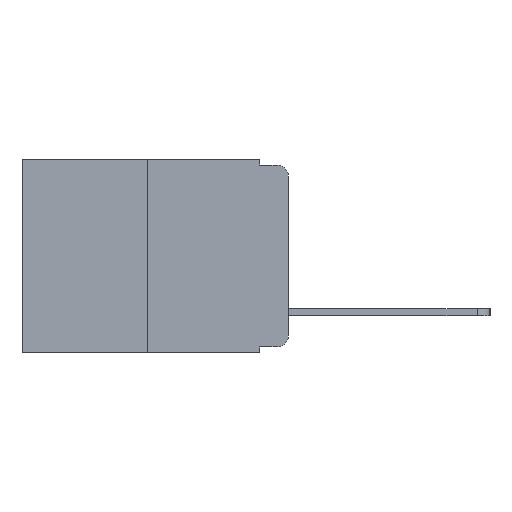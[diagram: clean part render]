
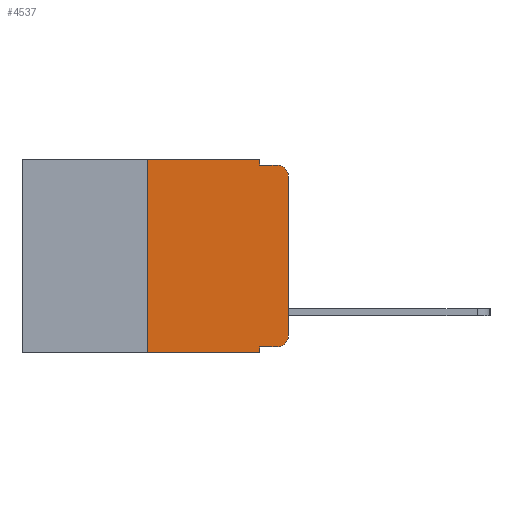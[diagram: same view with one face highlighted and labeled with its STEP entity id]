
A CAD part, left-side view. The second image highlights one B-rep face of the part: STEP entity #4537.
In plain terms, the highlighted planar face has unit normal (-1, 0, 0).
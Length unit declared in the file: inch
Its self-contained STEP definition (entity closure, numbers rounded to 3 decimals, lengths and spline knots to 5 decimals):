
#17 = CIRCLE ( 'NONE', #20758, 0.02 ) ;
#32 = VECTOR ( 'NONE', #8358, 39.37008 ) ;
#76 = DIRECTION ( 'NONE',  ( 0., -1., 0. ) ) ;
#261 = ORIENTED_EDGE ( 'NONE', *, *, #6416, .F. ) ;
#351 = VERTEX_POINT ( 'NONE', #8157 ) ;
#473 = VERTEX_POINT ( 'NONE', #11344 ) ;
#594 = CARTESIAN_POINT ( 'NONE',  ( 0., 0.051, 0. ) ) ;
#611 = AXIS2_PLACEMENT_3D ( 'NONE', #16874, #18416, #2044 ) ;
#669 = EDGE_CURVE ( 'NONE', #13733, #17383, #20309, .T. ) ;
#855 = CARTESIAN_POINT ( 'NONE',  ( 0., 0.25, 0. ) ) ;
#950 = DIRECTION ( 'NONE',  ( 0., 0., -1. ) ) ;
#1012 = VECTOR ( 'NONE', #12440, 39.37008 ) ;
#1279 = DIRECTION ( 'NONE',  ( 0., 0., -1. ) ) ;
#1845 = EDGE_CURVE ( 'NONE', #11778, #13733, #11550, .T. ) ;
#1929 = VERTEX_POINT ( 'NONE', #855 ) ;
#2044 = DIRECTION ( 'NONE',  ( 0., 0., -1. ) ) ;
#2176 = LINE ( 'NONE', #3964, #19258 ) ;
#2352 = DIRECTION ( 'NONE',  ( 0., -1., 0. ) ) ;
#2441 = VECTOR ( 'NONE', #18248, 39.37008 ) ;
#2777 = VECTOR ( 'NONE', #8556, 39.37008 ) ;
#2995 = VERTEX_POINT ( 'NONE', #15507 ) ;
#3964 = CARTESIAN_POINT ( 'NONE',  ( 0., 0.473, 0. ) ) ;
#4117 = EDGE_CURVE ( 'NONE', #11778, #473, #20318, .T. ) ;
#4208 = VECTOR ( 'NONE', #19559, 39.37008 ) ;
#4537 = ADVANCED_FACE ( 'NONE', ( #6743 ), #11356, .F. ) ;
#4577 = CARTESIAN_POINT ( 'NONE',  ( 0., 0.051, -0.01 ) ) ;
#5256 = EDGE_CURVE ( 'NONE', #351, #1929, #19521, .T. ) ;
#5560 = CARTESIAN_POINT ( 'NONE',  ( 0., 0.02, -0.333 ) ) ;
#5897 = CARTESIAN_POINT ( 'NONE',  ( 0., 0.051, 0. ) ) ;
#6416 = EDGE_CURVE ( 'NONE', #6516, #15698, #13912, .T. ) ;
#6516 = VERTEX_POINT ( 'NONE', #5897 ) ;
#6570 = VECTOR ( 'NONE', #76, 39.37008 ) ;
#6717 = EDGE_CURVE ( 'NONE', #351, #473, #8777, .T. ) ;
#6743 = FACE_OUTER_BOUND ( 'NONE', #13322, .T. ) ;
#6989 = ORIENTED_EDGE ( 'NONE', *, *, #1845, .T. ) ;
#8157 = CARTESIAN_POINT ( 'NONE',  ( 0., 0.25, -0.343 ) ) ;
#8338 = ORIENTED_EDGE ( 'NONE', *, *, #10920, .T. ) ;
#8358 = DIRECTION ( 'NONE',  ( 0., 0., 1. ) ) ;
#8556 = DIRECTION ( 'NONE',  ( 0., 0., -1. ) ) ;
#8717 = CARTESIAN_POINT ( 'NONE',  ( 0., 0.051, -0.01 ) ) ;
#8723 = EDGE_CURVE ( 'NONE', #15698, #11528, #13543, .T. ) ;
#8777 = LINE ( 'NONE', #21177, #4208 ) ;
#8848 = ORIENTED_EDGE ( 'NONE', *, *, #9826, .T. ) ;
#9166 = VECTOR ( 'NONE', #17813, 39.37008 ) ;
#9778 = CARTESIAN_POINT ( 'NONE',  ( 0., 0.473, 0. ) ) ;
#9826 = EDGE_CURVE ( 'NONE', #2995, #11528, #17, .T. ) ;
#10920 = EDGE_CURVE ( 'NONE', #17383, #2995, #12518, .T. ) ;
#11129 = DIRECTION ( 'NONE',  ( -1., 0., 0. ) ) ;
#11344 = CARTESIAN_POINT ( 'NONE',  ( 0., 0.051, -0.343 ) ) ;
#11356 = PLANE ( 'NONE',  #12160 ) ;
#11428 = DIRECTION ( 'NONE',  ( 1., 0., 0. ) ) ;
#11439 = ORIENTED_EDGE ( 'NONE', *, *, #669, .T. ) ;
#11528 = VERTEX_POINT ( 'NONE', #19815 ) ;
#11550 = LINE ( 'NONE', #17686, #6570 ) ;
#11778 = VERTEX_POINT ( 'NONE', #12328 ) ;
#12160 = AXIS2_PLACEMENT_3D ( 'NONE', #9778, #11428, #1279 ) ;
#12328 = CARTESIAN_POINT ( 'NONE',  ( 0., 0.051, -0.333 ) ) ;
#12440 = DIRECTION ( 'NONE',  ( 0., 0., -1. ) ) ;
#12518 = LINE ( 'NONE', #18091, #32 ) ;
#13238 = ORIENTED_EDGE ( 'NONE', *, *, #8723, .F. ) ;
#13322 = EDGE_LOOP ( 'NONE', ( #8338, #8848, #13238, #261, #14235, #18499, #14735, #19007, #6989, #11439 ) ) ;
#13543 = LINE ( 'NONE', #4577, #9166 ) ;
#13733 = VERTEX_POINT ( 'NONE', #5560 ) ;
#13912 = LINE ( 'NONE', #594, #1012 ) ;
#14235 = ORIENTED_EDGE ( 'NONE', *, *, #17984, .F. ) ;
#14735 = ORIENTED_EDGE ( 'NONE', *, *, #6717, .T. ) ;
#15124 = CARTESIAN_POINT ( 'NONE',  ( 0., 0.051, 0. ) ) ;
#15507 = CARTESIAN_POINT ( 'NONE',  ( 0., 0., -0.03 ) ) ;
#15698 = VERTEX_POINT ( 'NONE', #8717 ) ;
#16629 = CARTESIAN_POINT ( 'NONE',  ( 0., 0.25, 0. ) ) ;
#16874 = CARTESIAN_POINT ( 'NONE',  ( 0., 0.02, -0.313 ) ) ;
#17158 = CARTESIAN_POINT ( 'NONE',  ( 0., 0., -0.313 ) ) ;
#17383 = VERTEX_POINT ( 'NONE', #17158 ) ;
#17686 = CARTESIAN_POINT ( 'NONE',  ( 0., 0.051, -0.333 ) ) ;
#17813 = DIRECTION ( 'NONE',  ( 0., -1., 0. ) ) ;
#17984 = EDGE_CURVE ( 'NONE', #1929, #6516, #2176, .T. ) ;
#18091 = CARTESIAN_POINT ( 'NONE',  ( 0., 0., 0. ) ) ;
#18248 = DIRECTION ( 'NONE',  ( 0., 0., 1. ) ) ;
#18416 = DIRECTION ( 'NONE',  ( -1., 0., 0. ) ) ;
#18499 = ORIENTED_EDGE ( 'NONE', *, *, #5256, .F. ) ;
#19007 = ORIENTED_EDGE ( 'NONE', *, *, #4117, .F. ) ;
#19258 = VECTOR ( 'NONE', #2352, 39.37008 ) ;
#19521 = LINE ( 'NONE', #16629, #2441 ) ;
#19559 = DIRECTION ( 'NONE',  ( 0., -1., 0. ) ) ;
#19815 = CARTESIAN_POINT ( 'NONE',  ( 0., 0.02, -0.01 ) ) ;
#20309 = CIRCLE ( 'NONE', #611, 0.02 ) ;
#20318 = LINE ( 'NONE', #15124, #2777 ) ;
#20758 = AXIS2_PLACEMENT_3D ( 'NONE', #20805, #11129, #950 ) ;
#20805 = CARTESIAN_POINT ( 'NONE',  ( 0., 0.02, -0.03 ) ) ;
#21177 = CARTESIAN_POINT ( 'NONE',  ( 0., 0.473, -0.343 ) ) ;
